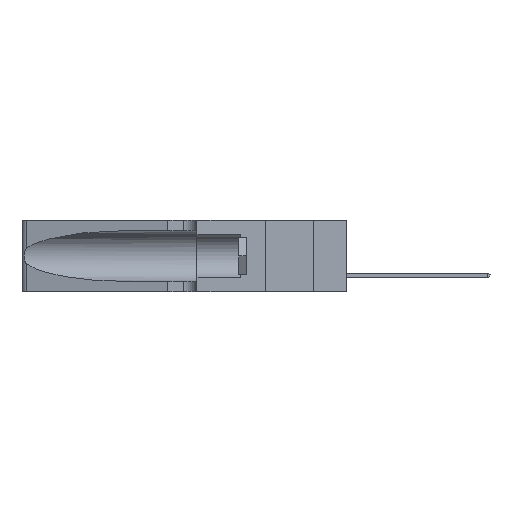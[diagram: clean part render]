
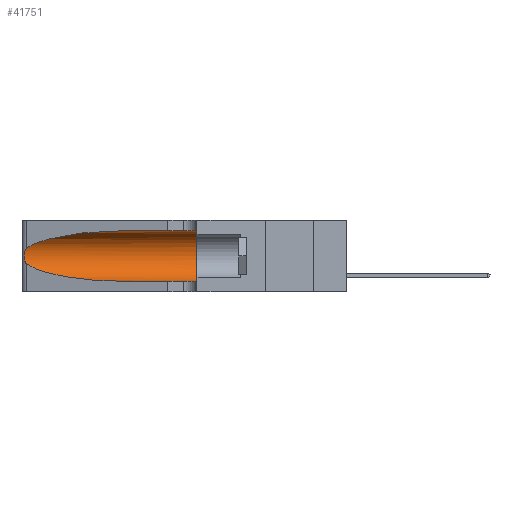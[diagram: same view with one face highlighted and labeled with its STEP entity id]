
A CAD part, left-side view. The second image highlights one B-rep face of the part: STEP entity #41751.
In plain terms, the highlighted cylindrical face has radius 3.308 mm (diameter 6.617 mm), a partial arc.
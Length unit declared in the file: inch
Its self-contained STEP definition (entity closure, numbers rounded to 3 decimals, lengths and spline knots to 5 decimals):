
#799 = VERTEX_POINT ( 'NONE', #36017 ) ;
#2980 = VECTOR ( 'NONE', #34834, 39.37008 ) ;
#4590 = VERTEX_POINT ( 'NONE', #18640 ) ;
#5517 = CARTESIAN_POINT ( 'NONE',  ( 0.26075, 1.23896, 0.178 ) ) ;
#5522 = CARTESIAN_POINT ( 'NONE',  ( 0.1305, 0.35, 0.185 ) ) ;
#6112 = CARTESIAN_POINT ( 'NONE',  ( 0.1305, 0.72297, 0.05475 ) ) ;
#6270 = CARTESIAN_POINT ( 'NONE',  ( 0.18966, 0.96281, 0.05475 ) ) ;
#6361 = DIRECTION ( 'NONE',  ( 0., 0., -1. ) ) ;
#6568 = DIRECTION ( 'NONE',  ( 0., -1., 0. ) ) ;
#7857 = CYLINDRICAL_SURFACE ( 'NONE', #12917, 0.13025 ) ;
#8403 = FACE_OUTER_BOUND ( 'NONE', #35558, .T. ) ;
#8838 = ORIENTED_EDGE ( 'NONE', *, *, #11591, .T. ) ;
#9624 = EDGE_CURVE ( 'NONE', #27501, #4590, #33170, .T. ) ;
#9760 = DIRECTION ( 'NONE',  ( 0., -1., 0. ) ) ;
#9954 = EDGE_CURVE ( 'NONE', #29773, #27501, #25244, .T. ) ;
#11591 = EDGE_CURVE ( 'NONE', #4590, #799, #36454, .T. ) ;
#11592 = CARTESIAN_POINT ( 'NONE',  ( 0.2373, 1.15595, 0.28018 ) ) ;
#12382 = CARTESIAN_POINT ( 'NONE',  ( 0.26017, 1.23833, 0.17102 ) ) ;
#12917 = AXIS2_PLACEMENT_3D ( 'NONE', #22900, #9760, #6361 ) ;
#13902 = LINE ( 'NONE', #16692, #21348 ) ;
#13981 = ORIENTED_EDGE ( 'NONE', *, *, #33443, .F. ) ;
#14840 = ORIENTED_EDGE ( 'NONE', *, *, #30713, .T. ) ;
#15778 = AXIS2_PLACEMENT_3D ( 'NONE', #5522, #22953, #29814 ) ;
#16692 = CARTESIAN_POINT ( 'NONE',  ( 0.1305, 1.61858, 0.05475 ) ) ;
#18640 = CARTESIAN_POINT ( 'NONE',  ( 0.25487, 1.22718, 0.14631 ) ) ;
#19237 = CARTESIAN_POINT ( 'NONE',  ( 0.25555, 1.22993, 0.14849 ) ) ;
#20517 = VERTEX_POINT ( 'NONE', #29658 ) ;
#21348 = VECTOR ( 'NONE', #6568, 39.37008 ) ;
#22508 = CARTESIAN_POINT ( 'NONE',  ( 0.25555, 1.22994, 0.2215 ) ) ;
#22900 = CARTESIAN_POINT ( 'NONE',  ( 0.1305, 1.61858, 0.185 ) ) ;
#22953 = DIRECTION ( 'NONE',  ( 0., 1., 0. ) ) ;
#25244 =( BOUNDED_CURVE ( )  B_SPLINE_CURVE ( 3, ( #41960, #41667, #11592, #35282 ),
 .UNSPECIFIED., .F., .T. ) 
 B_SPLINE_CURVE_WITH_KNOTS ( ( 4, 4 ),
 ( 1.5708, 2.84003 ),
 .UNSPECIFIED. ) 
 CURVE ( )  GEOMETRIC_REPRESENTATION_ITEM ( )  RATIONAL_B_SPLINE_CURVE ( ( 1., 0.87, 0.87, 1. ) ) 
 REPRESENTATION_ITEM ( '' )  );
#25926 = CARTESIAN_POINT ( 'NONE',  ( 0.25854, 1.2359, 0.20912 ) ) ;
#26072 = ORIENTED_EDGE ( 'NONE', *, *, #9624, .T. ) ;
#26744 = ORIENTED_EDGE ( 'NONE', *, *, #30572, .F. ) ;
#27501 = VERTEX_POINT ( 'NONE', #43619 ) ;
#29205 = CARTESIAN_POINT ( 'NONE',  ( 0.25787, 1.23484, 0.2124 ) ) ;
#29657 = CARTESIAN_POINT ( 'NONE',  ( 0.25639, 1.23186, 0.15144 ) ) ;
#29658 = CARTESIAN_POINT ( 'NONE',  ( 0.1305, 0.35, 0.05475 ) ) ;
#29773 = VERTEX_POINT ( 'NONE', #35081 ) ;
#29809 = CARTESIAN_POINT ( 'NONE',  ( 0.25856, 1.23593, 0.16098 ) ) ;
#29814 = DIRECTION ( 'NONE',  ( 0., 0., 1. ) ) ;
#30572 = EDGE_CURVE ( 'NONE', #39343, #20517, #41039, .T. ) ;
#30713 = EDGE_CURVE ( 'NONE', #799, #20517, #13902, .T. ) ;
#30761 = CARTESIAN_POINT ( 'NONE',  ( 0.1305, 0.35, 0.31525 ) ) ;
#31400 = CARTESIAN_POINT ( 'NONE',  ( 0.1305, 1.61858, 0.31525 ) ) ;
#33170 = B_SPLINE_CURVE_WITH_KNOTS ( 'NONE', 3,
 ( #39618, #22508, #36211, #29205, #25926, #36359, #36050, #5517, #12382, #29809, #36648, #29657, #19237, #43046 ),
 .UNSPECIFIED., .F., .F.,
 ( 4, 2, 2, 2, 2, 2, 4 ),
 ( 0., 0.00027, 0.00053, 0.00107, 0.0016, 0.00187, 0.00214 ),
 .UNSPECIFIED. ) ;
#33443 = EDGE_CURVE ( 'NONE', #29773, #39343, #41874, .T. ) ;
#33524 = CARTESIAN_POINT ( 'NONE',  ( 0.2373, 1.15595, 0.08982 ) ) ;
#34374 = ORIENTED_EDGE ( 'NONE', *, *, #9954, .T. ) ;
#34834 = DIRECTION ( 'NONE',  ( 0., -1., 0. ) ) ;
#35081 = CARTESIAN_POINT ( 'NONE',  ( 0.1305, 0.72297, 0.31525 ) ) ;
#35282 = CARTESIAN_POINT ( 'NONE',  ( 0.25487, 1.22718, 0.22369 ) ) ;
#35558 = EDGE_LOOP ( 'NONE', ( #34374, #26072, #8838, #14840, #26744, #13981 ) ) ;
#36017 = CARTESIAN_POINT ( 'NONE',  ( 0.1305, 0.72297, 0.05475 ) ) ;
#36050 = CARTESIAN_POINT ( 'NONE',  ( 0.26075, 1.23896, 0.19203 ) ) ;
#36211 = CARTESIAN_POINT ( 'NONE',  ( 0.25639, 1.23184, 0.21858 ) ) ;
#36359 = CARTESIAN_POINT ( 'NONE',  ( 0.26018, 1.23835, 0.19895 ) ) ;
#36454 =( BOUNDED_CURVE ( )  B_SPLINE_CURVE ( 3, ( #43794, #33524, #6270, #6112 ),
 .UNSPECIFIED., .F., .T. ) 
 B_SPLINE_CURVE_WITH_KNOTS ( ( 4, 4 ),
 ( 3.44316, 4.71239 ),
 .UNSPECIFIED. ) 
 CURVE ( )  GEOMETRIC_REPRESENTATION_ITEM ( )  RATIONAL_B_SPLINE_CURVE ( ( 1., 0.87, 0.87, 1. ) ) 
 REPRESENTATION_ITEM ( '' )  );
#36648 = CARTESIAN_POINT ( 'NONE',  ( 0.25789, 1.23486, 0.15765 ) ) ;
#39343 = VERTEX_POINT ( 'NONE', #30761 ) ;
#39618 = CARTESIAN_POINT ( 'NONE',  ( 0.25487, 1.22718, 0.22369 ) ) ;
#41039 = CIRCLE ( 'NONE', #15778, 0.13025 ) ;
#41667 = CARTESIAN_POINT ( 'NONE',  ( 0.18966, 0.96281, 0.31525 ) ) ;
#41751 = ADVANCED_FACE ( 'NONE', ( #8403 ), #7857, .F. ) ;
#41874 = LINE ( 'NONE', #31400, #2980 ) ;
#41960 = CARTESIAN_POINT ( 'NONE',  ( 0.1305, 0.72297, 0.31525 ) ) ;
#43046 = CARTESIAN_POINT ( 'NONE',  ( 0.25487, 1.22718, 0.14631 ) ) ;
#43619 = CARTESIAN_POINT ( 'NONE',  ( 0.25487, 1.22718, 0.22369 ) ) ;
#43794 = CARTESIAN_POINT ( 'NONE',  ( 0.25487, 1.22718, 0.14631 ) ) ;
